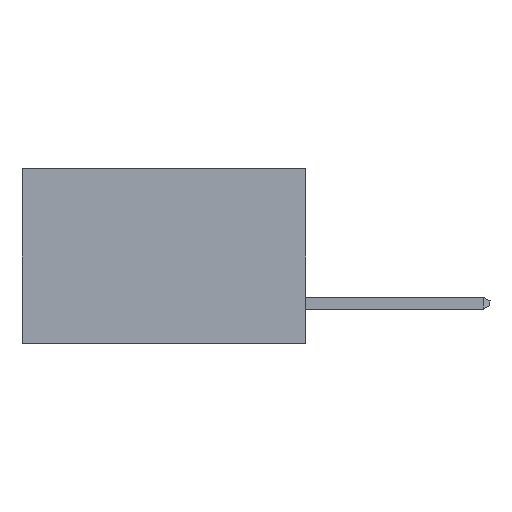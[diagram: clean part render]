
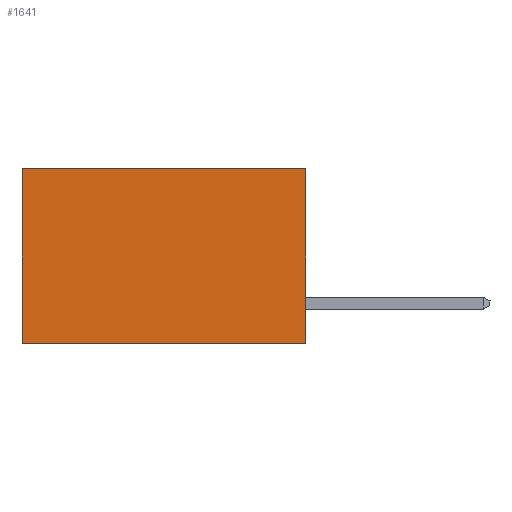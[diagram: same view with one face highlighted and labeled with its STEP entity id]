
A CAD part, left-side view. The second image highlights one B-rep face of the part: STEP entity #1641.
In plain terms, the highlighted planar face has unit normal (-1, 0, 0).
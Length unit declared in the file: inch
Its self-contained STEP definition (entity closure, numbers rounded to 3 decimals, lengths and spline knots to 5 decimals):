
#714 = DIRECTION ( 'NONE',  ( 0., 0., -1. ) ) ;
#798 = VERTEX_POINT ( 'NONE', #1856 ) ;
#1641 = ADVANCED_FACE ( 'NONE', ( #4414 ), #8363, .F. ) ;
#1794 = CARTESIAN_POINT ( 'NONE',  ( 0.2615, 0., -0.37 ) ) ;
#1856 = CARTESIAN_POINT ( 'NONE',  ( 0.2615, 0.6, -0.37 ) ) ;
#2862 = DIRECTION ( 'NONE',  ( 0., 1., 0. ) ) ;
#3285 = CARTESIAN_POINT ( 'NONE',  ( 0.2615, 0.6, 0. ) ) ;
#3805 = VECTOR ( 'NONE', #2862, 39.37008 ) ;
#4158 = AXIS2_PLACEMENT_3D ( 'NONE', #1794, #10615, #14422 ) ;
#4281 = ORIENTED_EDGE ( 'NONE', *, *, #11191, .T. ) ;
#4334 = DIRECTION ( 'NONE',  ( 0., 1., 0. ) ) ;
#4410 = VERTEX_POINT ( 'NONE', #8484 ) ;
#4414 = FACE_OUTER_BOUND ( 'NONE', #14083, .T. ) ;
#4901 = VECTOR ( 'NONE', #11208, 39.37008 ) ;
#4956 = VERTEX_POINT ( 'NONE', #15000 ) ;
#6817 = VECTOR ( 'NONE', #4334, 39.37008 ) ;
#6823 = CARTESIAN_POINT ( 'NONE',  ( 0.2615, 0., -0.37 ) ) ;
#7410 = ORIENTED_EDGE ( 'NONE', *, *, #9196, .F. ) ;
#7806 = LINE ( 'NONE', #14181, #3805 ) ;
#8363 = PLANE ( 'NONE',  #4158 ) ;
#8484 = CARTESIAN_POINT ( 'NONE',  ( 0.2615, 0., -0.37 ) ) ;
#8643 = ORIENTED_EDGE ( 'NONE', *, *, #9384, .T. ) ;
#9196 = EDGE_CURVE ( 'NONE', #4956, #4410, #12379, .T. ) ;
#9384 = EDGE_CURVE ( 'NONE', #4956, #14387, #7806, .T. ) ;
#10615 = DIRECTION ( 'NONE',  ( 1., 0., 0. ) ) ;
#10989 = VECTOR ( 'NONE', #714, 39.37008 ) ;
#11191 = EDGE_CURVE ( 'NONE', #14387, #798, #14492, .T. ) ;
#11208 = DIRECTION ( 'NONE',  ( 0., 0., -1. ) ) ;
#12022 = CARTESIAN_POINT ( 'NONE',  ( 0.2615, 0.6, -0.37 ) ) ;
#12379 = LINE ( 'NONE', #16074, #4901 ) ;
#13650 = EDGE_CURVE ( 'NONE', #4410, #798, #15649, .T. ) ;
#14083 = EDGE_LOOP ( 'NONE', ( #4281, #14811, #7410, #8643 ) ) ;
#14181 = CARTESIAN_POINT ( 'NONE',  ( 0.2615, 0., 0. ) ) ;
#14387 = VERTEX_POINT ( 'NONE', #3285 ) ;
#14422 = DIRECTION ( 'NONE',  ( 0., 0., -1. ) ) ;
#14492 = LINE ( 'NONE', #12022, #10989 ) ;
#14811 = ORIENTED_EDGE ( 'NONE', *, *, #13650, .F. ) ;
#15000 = CARTESIAN_POINT ( 'NONE',  ( 0.2615, 0., 0. ) ) ;
#15649 = LINE ( 'NONE', #6823, #6817 ) ;
#16074 = CARTESIAN_POINT ( 'NONE',  ( 0.2615, 0., -0.37 ) ) ;
